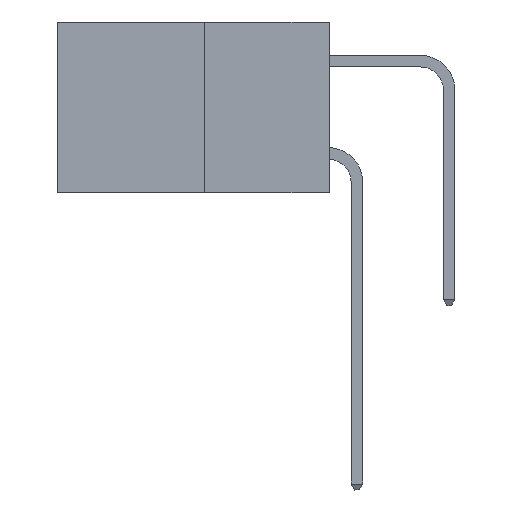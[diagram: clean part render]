
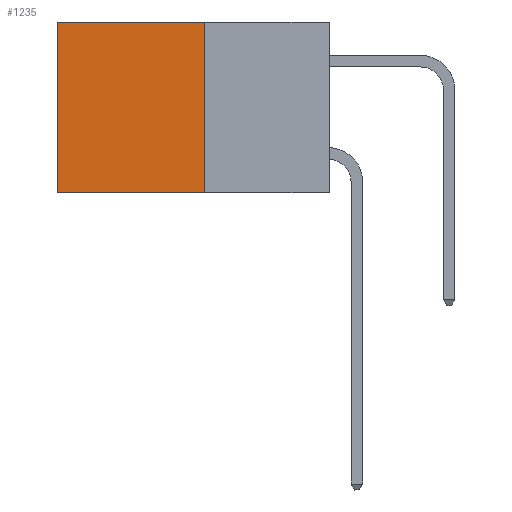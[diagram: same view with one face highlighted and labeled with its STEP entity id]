
A CAD part, left-side view. The second image highlights one B-rep face of the part: STEP entity #1235.
In plain terms, the highlighted planar face has unit normal (-1, 0, 0).
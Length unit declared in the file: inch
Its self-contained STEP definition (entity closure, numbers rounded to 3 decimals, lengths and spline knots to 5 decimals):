
#184 = EDGE_LOOP ( 'NONE', ( #1876, #5427, #6015, #3899 ) ) ;
#1235 = ADVANCED_FACE ( 'NONE', ( #11614 ), #1382, .F. ) ;
#1382 = PLANE ( 'NONE',  #10766 ) ;
#1598 = CARTESIAN_POINT ( 'NONE',  ( 0.277, 0.59, -0.37 ) ) ;
#1850 = DIRECTION ( 'NONE',  ( 0., 0., -1. ) ) ;
#1876 = ORIENTED_EDGE ( 'NONE', *, *, #4804, .T. ) ;
#2169 = VERTEX_POINT ( 'NONE', #1598 ) ;
#3644 = VERTEX_POINT ( 'NONE', #5801 ) ;
#3899 = ORIENTED_EDGE ( 'NONE', *, *, #11302, .T. ) ;
#3990 = CARTESIAN_POINT ( 'NONE',  ( 0.277, 0.27, -0.37 ) ) ;
#4258 = VERTEX_POINT ( 'NONE', #5905 ) ;
#4804 = EDGE_CURVE ( 'NONE', #9924, #2169, #8838, .T. ) ;
#5427 = ORIENTED_EDGE ( 'NONE', *, *, #11142, .F. ) ;
#5732 = LINE ( 'NONE', #3990, #8156 ) ;
#5801 = CARTESIAN_POINT ( 'NONE',  ( 0.277, 0.27, -0.37 ) ) ;
#5905 = CARTESIAN_POINT ( 'NONE',  ( 0.277, 0.27, 0. ) ) ;
#6015 = ORIENTED_EDGE ( 'NONE', *, *, #7180, .F. ) ;
#6384 = CARTESIAN_POINT ( 'NONE',  ( 0.277, 0.27, -0.37 ) ) ;
#6778 = VECTOR ( 'NONE', #1850, 39.37008 ) ;
#6899 = DIRECTION ( 'NONE',  ( 0., 1., 0. ) ) ;
#7180 = EDGE_CURVE ( 'NONE', #4258, #3644, #9239, .T. ) ;
#7398 = LINE ( 'NONE', #8761, #9879 ) ;
#8156 = VECTOR ( 'NONE', #8507, 39.37008 ) ;
#8180 = CARTESIAN_POINT ( 'NONE',  ( 0.277, 0.27, -0.37 ) ) ;
#8507 = DIRECTION ( 'NONE',  ( 0., 1., 0. ) ) ;
#8761 = CARTESIAN_POINT ( 'NONE',  ( 0.277, 0.27, 0. ) ) ;
#8838 = LINE ( 'NONE', #9913, #10934 ) ;
#9239 = LINE ( 'NONE', #8180, #6778 ) ;
#9879 = VECTOR ( 'NONE', #6899, 39.37008 ) ;
#9900 = DIRECTION ( 'NONE',  ( 0., 0., -1. ) ) ;
#9913 = CARTESIAN_POINT ( 'NONE',  ( 0.277, 0.59, -0.37 ) ) ;
#9924 = VERTEX_POINT ( 'NONE', #11715 ) ;
#10579 = DIRECTION ( 'NONE',  ( 1., 0., 0. ) ) ;
#10766 = AXIS2_PLACEMENT_3D ( 'NONE', #6384, #10579, #9900 ) ;
#10782 = DIRECTION ( 'NONE',  ( 0., 0., -1. ) ) ;
#10934 = VECTOR ( 'NONE', #10782, 39.37008 ) ;
#11142 = EDGE_CURVE ( 'NONE', #3644, #2169, #5732, .T. ) ;
#11302 = EDGE_CURVE ( 'NONE', #4258, #9924, #7398, .T. ) ;
#11614 = FACE_OUTER_BOUND ( 'NONE', #184, .T. ) ;
#11715 = CARTESIAN_POINT ( 'NONE',  ( 0.277, 0.59, 0. ) ) ;
